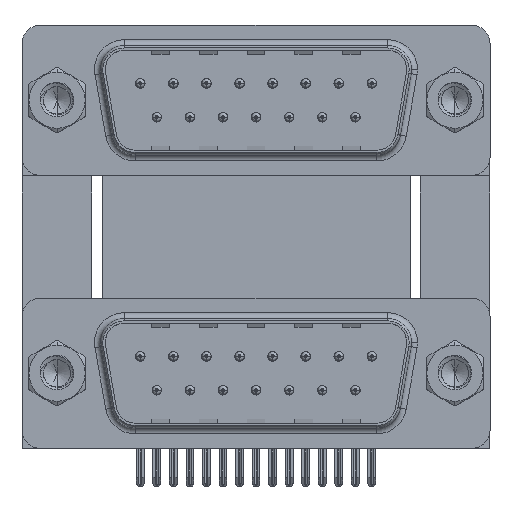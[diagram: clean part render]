
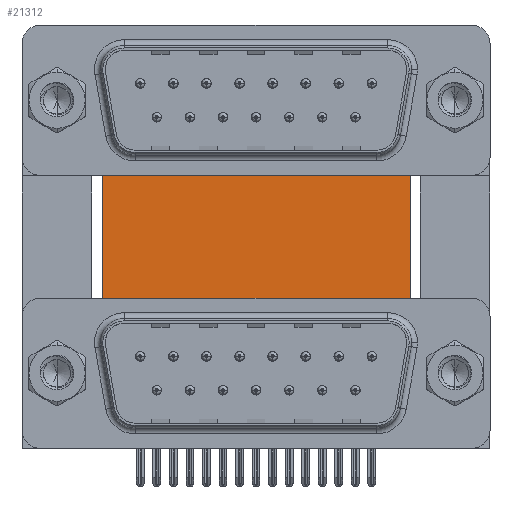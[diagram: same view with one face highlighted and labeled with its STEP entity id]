
A CAD part, top view. The second image highlights one B-rep face of the part: STEP entity #21312.
In plain terms, the highlighted planar face has unit normal (0, 0, 1).
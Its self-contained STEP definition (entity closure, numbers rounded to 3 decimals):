
#1306 = VERTEX_POINT ( 'NONE', #28781 ) ;
#1744 = CARTESIAN_POINT ( 'NONE',  ( 3.79, -3.735, -12. ) ) ;
#3323 = CARTESIAN_POINT ( 'NONE',  ( 3.79, 16.585, -12. ) ) ;
#5926 = LINE ( 'NONE', #17096, #20662 ) ;
#6316 = LINE ( 'NONE', #17497, #26568 ) ;
#6934 = DIRECTION ( 'NONE',  ( 0., 0., -1. ) ) ;
#7013 = EDGE_CURVE ( 'NONE', #20767, #12271, #8563, .T. ) ;
#7151 = VERTEX_POINT ( 'NONE', #17025 ) ;
#7880 = ORIENTED_EDGE ( 'NONE', *, *, #23293, .F. ) ;
#8534 = VECTOR ( 'NONE', #33670, 1000. ) ;
#8563 = LINE ( 'NONE', #19738, #8534 ) ;
#9670 = DIRECTION ( 'NONE',  ( -1., 0., 0. ) ) ;
#11588 = VECTOR ( 'NONE', #22902, 1000. ) ;
#12271 = VERTEX_POINT ( 'NONE', #1744 ) ;
#12553 = EDGE_CURVE ( 'NONE', #20767, #7151, #20524, .T. ) ;
#12616 = FACE_OUTER_BOUND ( 'NONE', #13344, .T. ) ;
#13344 = EDGE_LOOP ( 'NONE', ( #15397, #7880, #35529, #19361 ) ) ;
#15397 = ORIENTED_EDGE ( 'NONE', *, *, #33599, .T. ) ;
#17025 = CARTESIAN_POINT ( 'NONE',  ( 29.58, 16.585, -12. ) ) ;
#17096 = CARTESIAN_POINT ( 'NONE',  ( 3.79, -3.735, -12. ) ) ;
#17497 = CARTESIAN_POINT ( 'NONE',  ( 29.58, 16.585, -12. ) ) ;
#17936 = PLANE ( 'NONE',  #28163 ) ;
#19361 = ORIENTED_EDGE ( 'NONE', *, *, #7013, .T. ) ;
#19738 = CARTESIAN_POINT ( 'NONE',  ( 3.79, 16.585, -12. ) ) ;
#20524 = LINE ( 'NONE', #3323, #11588 ) ;
#20662 = VECTOR ( 'NONE', #25866, 1000. ) ;
#20767 = VERTEX_POINT ( 'NONE', #28859 ) ;
#21312 = ADVANCED_FACE ( 'NONE', ( #12616 ), #17936, .F. ) ;
#22902 = DIRECTION ( 'NONE',  ( 1., 0., 0. ) ) ;
#23232 = CARTESIAN_POINT ( 'NONE',  ( 3.79, 16.585, -12. ) ) ;
#23293 = EDGE_CURVE ( 'NONE', #7151, #1306, #6316, .T. ) ;
#25866 = DIRECTION ( 'NONE',  ( 1., 0., 0. ) ) ;
#26568 = VECTOR ( 'NONE', #28647, 1000. ) ;
#28163 = AXIS2_PLACEMENT_3D ( 'NONE', #23232, #6934, #9670 ) ;
#28647 = DIRECTION ( 'NONE',  ( 0., -1., 0. ) ) ;
#28781 = CARTESIAN_POINT ( 'NONE',  ( 29.58, -3.735, -12. ) ) ;
#28859 = CARTESIAN_POINT ( 'NONE',  ( 3.79, 16.585, -12. ) ) ;
#33599 = EDGE_CURVE ( 'NONE', #12271, #1306, #5926, .T. ) ;
#33670 = DIRECTION ( 'NONE',  ( 0., -1., 0. ) ) ;
#35529 = ORIENTED_EDGE ( 'NONE', *, *, #12553, .F. ) ;
